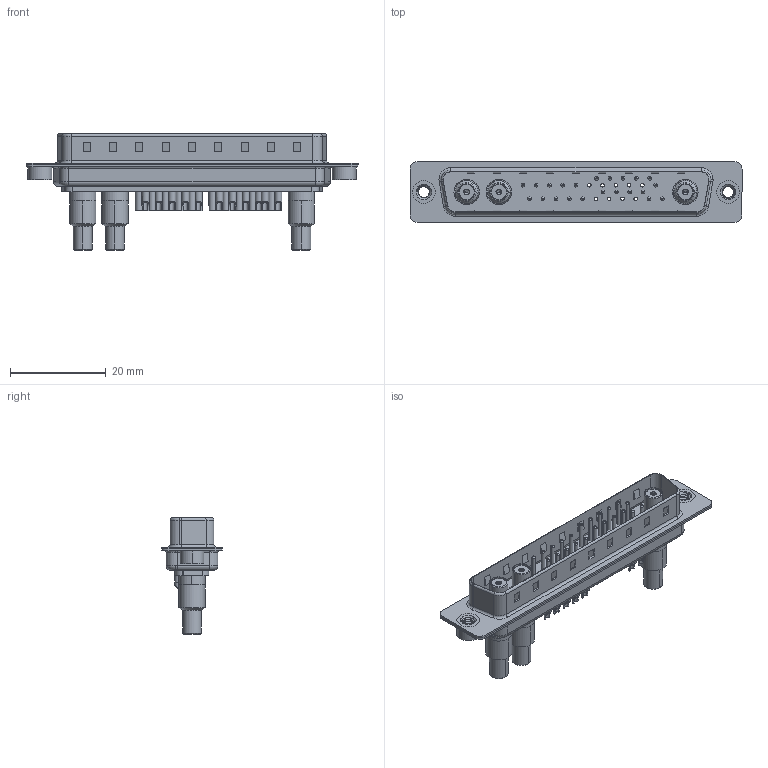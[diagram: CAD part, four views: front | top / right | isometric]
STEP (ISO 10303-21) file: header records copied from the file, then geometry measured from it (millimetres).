
FILE_DESCRIPTION (( 'STEP AP203' ), '1' );
FILE_NAME ('627-25W3222-5NA.STEP', '2019-05-29T09:00:51', ( '' ), ( '' ), 'SwSTEP 2.0', 'SolidWorks 2016', '' );
FILE_SCHEMA (( 'CONFIG_CONTROL_DESIGN' ));
Length unit declared in the file: millimetre
Products named in the file (15): Socket_Solder Cup; 627Combo Housing_25W3; Solder Cover; 627Combo Shell Rear_37 Contacts; Co-Ax Jack Assy_SC; 627Combo Shell Front_37 Contacts; 627Combo Threaded Rivet_2; 627Combo Threaded Rivet_A; 627Combo Contact Row 1_22; Co-Ax Jack_Solder Cup Tail; 627Combo Contact Row 2_22; Insulator Socket; 627-25W3222-5NA; Insulator Socket 2; Locking Collar
Assembly tree (36 placements, depth 3):
  627-25W3222-5NA
    627Combo Housing_25W3
    627Combo Shell Rear_37 Contacts
    627Combo Shell Front_37 Contacts
    627Combo Threaded Rivet_A
    Co-Ax Jack Assy_SC  x3
      Co-Ax Jack_Solder Cup Tail
      Insulator Socket
      Insulator Socket 2
      Locking Collar
      Socket_Solder Cup
      Solder Cover
    627Combo Threaded Rivet_2
    627Combo Contact Row 1_22  x11
    627Combo Contact Row 2_22  x11
Bounding box: 69.3 x 12.6 x 24.3 mm (x, y, z)
Volume: 4183.7 mm3; surface area: 11863.4 mm2
Topology: 45 solids, 45 shells, 1615 faces, 3769 edges, 2314 vertices
Faces by surface type: cylinder 686, plane 521, torus 282, cone 114, bspline 12
Entity records: 28676 total; most frequent: CARTESIAN_POINT 7452, DIRECTION 4227, ORIENTED_EDGE 3770, EDGE_CURVE 1885, AXIS2_PLACEMENT_3D 1638, VERTEX_POINT 1198, EDGE_LOOP 969, VECTOR 951
